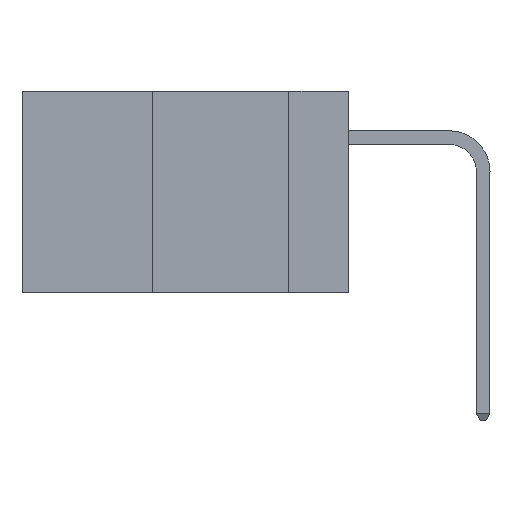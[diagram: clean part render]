
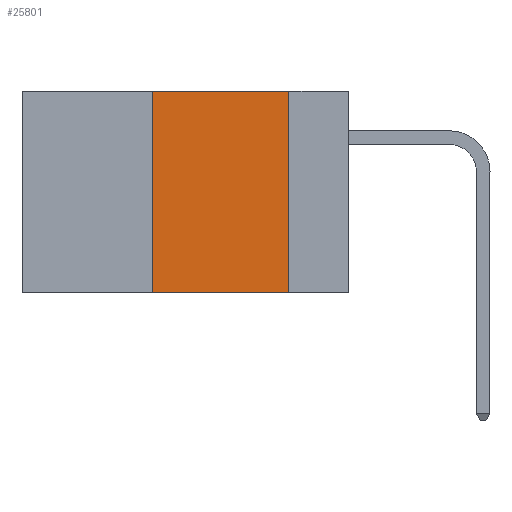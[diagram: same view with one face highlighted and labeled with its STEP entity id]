
A CAD part, left-side view. The second image highlights one B-rep face of the part: STEP entity #25801.
In plain terms, the highlighted planar face has unit normal (-1, 0, 0).
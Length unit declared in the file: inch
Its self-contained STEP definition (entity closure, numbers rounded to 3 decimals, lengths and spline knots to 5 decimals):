
#2333 = DIRECTION ( 'NONE',  ( 0., 0., 1. ) ) ;
#5362 = ORIENTED_EDGE ( 'NONE', *, *, #33782, .F. ) ;
#8863 = PLANE ( 'NONE',  #18601 ) ;
#8995 = DIRECTION ( 'NONE',  ( 1., 0., 0. ) ) ;
#9400 = VERTEX_POINT ( 'NONE', #21586 ) ;
#12272 = EDGE_CURVE ( 'NONE', #16540, #35309, #35469, .T. ) ;
#12340 = CARTESIAN_POINT ( 'NONE',  ( 0., 0.11, 0. ) ) ;
#12679 = VECTOR ( 'NONE', #25882, 39.37008 ) ;
#12693 = LINE ( 'NONE', #32723, #28882 ) ;
#12759 = LINE ( 'NONE', #34096, #20440 ) ;
#16500 = VERTEX_POINT ( 'NONE', #18846 ) ;
#16540 = VERTEX_POINT ( 'NONE', #21965 ) ;
#18601 = AXIS2_PLACEMENT_3D ( 'NONE', #26274, #8995, #29142 ) ;
#18846 = CARTESIAN_POINT ( 'NONE',  ( 0., 0.36, -0.37 ) ) ;
#20440 = VECTOR ( 'NONE', #2333, 39.37008 ) ;
#21209 = ORIENTED_EDGE ( 'NONE', *, *, #12272, .F. ) ;
#21409 = DIRECTION ( 'NONE',  ( 0., -1., 0. ) ) ;
#21586 = CARTESIAN_POINT ( 'NONE',  ( 0., 0.11, -0.37 ) ) ;
#21965 = CARTESIAN_POINT ( 'NONE',  ( 0., 0.36, 0. ) ) ;
#25383 = ORIENTED_EDGE ( 'NONE', *, *, #35421, .T. ) ;
#25801 = ADVANCED_FACE ( 'NONE', ( #25872 ), #8863, .F. ) ;
#25872 = FACE_OUTER_BOUND ( 'NONE', #34598, .T. ) ;
#25882 = DIRECTION ( 'NONE',  ( 0., -1., 0. ) ) ;
#25923 = VECTOR ( 'NONE', #34479, 39.37008 ) ;
#26274 = CARTESIAN_POINT ( 'NONE',  ( 0., 0.6, 0. ) ) ;
#28786 = CARTESIAN_POINT ( 'NONE',  ( 0., 0.11, 0. ) ) ;
#28882 = VECTOR ( 'NONE', #21409, 39.37008 ) ;
#29142 = DIRECTION ( 'NONE',  ( 0., 0., -1. ) ) ;
#31507 = ORIENTED_EDGE ( 'NONE', *, *, #32130, .F. ) ;
#32130 = EDGE_CURVE ( 'NONE', #35309, #9400, #33474, .T. ) ;
#32723 = CARTESIAN_POINT ( 'NONE',  ( 0., 0.6, -0.37 ) ) ;
#33474 = LINE ( 'NONE', #28786, #25923 ) ;
#33782 = EDGE_CURVE ( 'NONE', #16500, #16540, #12759, .T. ) ;
#34096 = CARTESIAN_POINT ( 'NONE',  ( 0., 0.36, 0. ) ) ;
#34479 = DIRECTION ( 'NONE',  ( 0., 0., -1. ) ) ;
#34598 = EDGE_LOOP ( 'NONE', ( #31507, #21209, #5362, #25383 ) ) ;
#35309 = VERTEX_POINT ( 'NONE', #12340 ) ;
#35421 = EDGE_CURVE ( 'NONE', #16500, #9400, #12693, .T. ) ;
#35469 = LINE ( 'NONE', #37263, #12679 ) ;
#37263 = CARTESIAN_POINT ( 'NONE',  ( 0., 0.6, 0. ) ) ;
